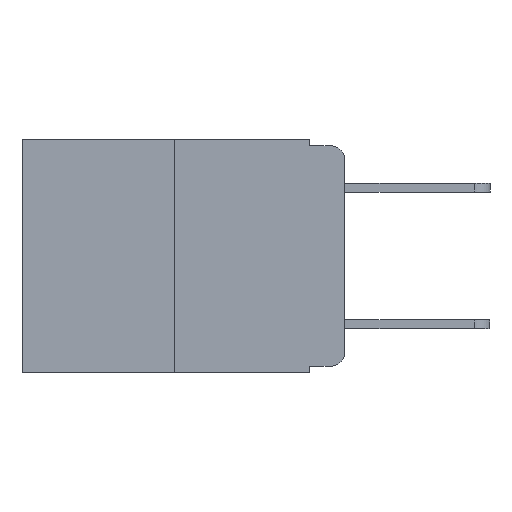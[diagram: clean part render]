
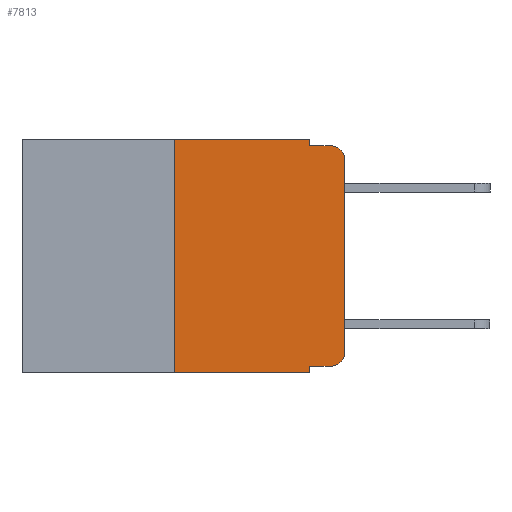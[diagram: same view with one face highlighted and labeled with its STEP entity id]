
A CAD part, left-side view. The second image highlights one B-rep face of the part: STEP entity #7813.
In plain terms, the highlighted planar face has unit normal (-1, 0, 0).
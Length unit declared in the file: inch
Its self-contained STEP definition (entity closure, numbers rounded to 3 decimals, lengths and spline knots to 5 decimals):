
#6 = EDGE_CURVE ( 'NONE', #21872, #60, #21228, .T. ) ;
#60 = VERTEX_POINT ( 'NONE', #10040 ) ;
#69 = CARTESIAN_POINT ( 'NONE',  ( 0., 0.473, 0. ) ) ;
#152 = DIRECTION ( 'NONE',  ( 1., 0., 0. ) ) ;
#165 = EDGE_CURVE ( 'NONE', #21872, #1309, #4648, .T. ) ;
#836 = VERTEX_POINT ( 'NONE', #17662 ) ;
#857 = ORIENTED_EDGE ( 'NONE', *, *, #3164, .T. ) ;
#1309 = VERTEX_POINT ( 'NONE', #5958 ) ;
#1410 = EDGE_LOOP ( 'NONE', ( #857, #10851, #14489, #15043, #17533, #13911, #21630, #7935, #15850, #1774 ) ) ;
#1774 = ORIENTED_EDGE ( 'NONE', *, *, #23021, .T. ) ;
#2970 = CARTESIAN_POINT ( 'NONE',  ( 0., 0.473, -0.343 ) ) ;
#3164 = EDGE_CURVE ( 'NONE', #22611, #7104, #9164, .T. ) ;
#3656 = EDGE_CURVE ( 'NONE', #12401, #17420, #13941, .T. ) ;
#3920 = DIRECTION ( 'NONE',  ( 0., -1., 0. ) ) ;
#4241 = VECTOR ( 'NONE', #17035, 39.37008 ) ;
#4648 = LINE ( 'NONE', #8524, #13777 ) ;
#5312 = CARTESIAN_POINT ( 'NONE',  ( 0., 0.051, -0.01 ) ) ;
#5614 = AXIS2_PLACEMENT_3D ( 'NONE', #6951, #19510, #8801 ) ;
#5806 = EDGE_CURVE ( 'NONE', #15143, #836, #20633, .T. ) ;
#5958 = CARTESIAN_POINT ( 'NONE',  ( 0., 0.25, 0. ) ) ;
#6156 = CARTESIAN_POINT ( 'NONE',  ( 0., 0.051, 0. ) ) ;
#6412 = DIRECTION ( 'NONE',  ( 0., 0., -1. ) ) ;
#6481 = DIRECTION ( 'NONE',  ( 0., -1., 0. ) ) ;
#6951 = CARTESIAN_POINT ( 'NONE',  ( 0., 0.02, -0.313 ) ) ;
#7104 = VERTEX_POINT ( 'NONE', #9035 ) ;
#7767 = CARTESIAN_POINT ( 'NONE',  ( 0., 0.473, 0. ) ) ;
#7813 = ADVANCED_FACE ( 'NONE', ( #21923 ), #11407, .F. ) ;
#7935 = ORIENTED_EDGE ( 'NONE', *, *, #19090, .F. ) ;
#7978 = DIRECTION ( 'NONE',  ( -1., 0., 0. ) ) ;
#8055 = VECTOR ( 'NONE', #9619, 39.37008 ) ;
#8524 = CARTESIAN_POINT ( 'NONE',  ( 0., 0.25, 0. ) ) ;
#8585 = EDGE_CURVE ( 'NONE', #7104, #8638, #20814, .T. ) ;
#8638 = VERTEX_POINT ( 'NONE', #11740 ) ;
#8652 = LINE ( 'NONE', #7767, #8055 ) ;
#8801 = DIRECTION ( 'NONE',  ( 0., 0., -1. ) ) ;
#9035 = CARTESIAN_POINT ( 'NONE',  ( 0., 0., -0.03 ) ) ;
#9090 = CIRCLE ( 'NONE', #5614, 0.02 ) ;
#9164 = LINE ( 'NONE', #12828, #18691 ) ;
#9381 = CARTESIAN_POINT ( 'NONE',  ( 0., 0., -0.313 ) ) ;
#9619 = DIRECTION ( 'NONE',  ( 0., -1., 0. ) ) ;
#9693 = CARTESIAN_POINT ( 'NONE',  ( 0., 0.051, -0.01 ) ) ;
#10040 = CARTESIAN_POINT ( 'NONE',  ( 0., 0.051, -0.343 ) ) ;
#10851 = ORIENTED_EDGE ( 'NONE', *, *, #8585, .T. ) ;
#11407 = PLANE ( 'NONE',  #14989 ) ;
#11492 = EDGE_CURVE ( 'NONE', #17420, #8638, #16591, .T. ) ;
#11588 = CARTESIAN_POINT ( 'NONE',  ( 0., 0.051, 0. ) ) ;
#11740 = CARTESIAN_POINT ( 'NONE',  ( 0., 0.02, -0.01 ) ) ;
#11819 = VECTOR ( 'NONE', #18128, 39.37008 ) ;
#11868 = VECTOR ( 'NONE', #6412, 39.37008 ) ;
#12304 = EDGE_CURVE ( 'NONE', #1309, #12401, #8652, .T. ) ;
#12401 = VERTEX_POINT ( 'NONE', #6156 ) ;
#12828 = CARTESIAN_POINT ( 'NONE',  ( 0., 0., 0. ) ) ;
#13201 = DIRECTION ( 'NONE',  ( 0., 0., -1. ) ) ;
#13501 = DIRECTION ( 'NONE',  ( 0., 0., 1. ) ) ;
#13777 = VECTOR ( 'NONE', #21449, 39.37008 ) ;
#13911 = ORIENTED_EDGE ( 'NONE', *, *, #165, .F. ) ;
#13941 = LINE ( 'NONE', #11588, #4241 ) ;
#14489 = ORIENTED_EDGE ( 'NONE', *, *, #11492, .F. ) ;
#14989 = AXIS2_PLACEMENT_3D ( 'NONE', #69, #152, #13201 ) ;
#15043 = ORIENTED_EDGE ( 'NONE', *, *, #3656, .F. ) ;
#15143 = VERTEX_POINT ( 'NONE', #16477 ) ;
#15850 = ORIENTED_EDGE ( 'NONE', *, *, #5806, .T. ) ;
#16477 = CARTESIAN_POINT ( 'NONE',  ( 0., 0.051, -0.333 ) ) ;
#16495 = AXIS2_PLACEMENT_3D ( 'NONE', #18767, #7978, #20492 ) ;
#16589 = VECTOR ( 'NONE', #6481, 39.37008 ) ;
#16591 = LINE ( 'NONE', #5312, #11819 ) ;
#16647 = LINE ( 'NONE', #17236, #11868 ) ;
#17035 = DIRECTION ( 'NONE',  ( 0., 0., -1. ) ) ;
#17236 = CARTESIAN_POINT ( 'NONE',  ( 0., 0.051, 0. ) ) ;
#17420 = VERTEX_POINT ( 'NONE', #9693 ) ;
#17533 = ORIENTED_EDGE ( 'NONE', *, *, #12304, .F. ) ;
#17662 = CARTESIAN_POINT ( 'NONE',  ( 0., 0.02, -0.333 ) ) ;
#18128 = DIRECTION ( 'NONE',  ( 0., -1., 0. ) ) ;
#18691 = VECTOR ( 'NONE', #13501, 39.37008 ) ;
#18767 = CARTESIAN_POINT ( 'NONE',  ( 0., 0.02, -0.03 ) ) ;
#19090 = EDGE_CURVE ( 'NONE', #15143, #60, #16647, .T. ) ;
#19510 = DIRECTION ( 'NONE',  ( -1., 0., 0. ) ) ;
#20067 = CARTESIAN_POINT ( 'NONE',  ( 0., 0.051, -0.333 ) ) ;
#20090 = VECTOR ( 'NONE', #3920, 39.37008 ) ;
#20492 = DIRECTION ( 'NONE',  ( 0., 0., -1. ) ) ;
#20633 = LINE ( 'NONE', #20067, #20090 ) ;
#20814 = CIRCLE ( 'NONE', #16495, 0.02 ) ;
#21146 = CARTESIAN_POINT ( 'NONE',  ( 0., 0.25, -0.343 ) ) ;
#21228 = LINE ( 'NONE', #2970, #16589 ) ;
#21449 = DIRECTION ( 'NONE',  ( 0., 0., 1. ) ) ;
#21630 = ORIENTED_EDGE ( 'NONE', *, *, #6, .T. ) ;
#21872 = VERTEX_POINT ( 'NONE', #21146 ) ;
#21923 = FACE_OUTER_BOUND ( 'NONE', #1410, .T. ) ;
#22611 = VERTEX_POINT ( 'NONE', #9381 ) ;
#23021 = EDGE_CURVE ( 'NONE', #836, #22611, #9090, .T. ) ;
